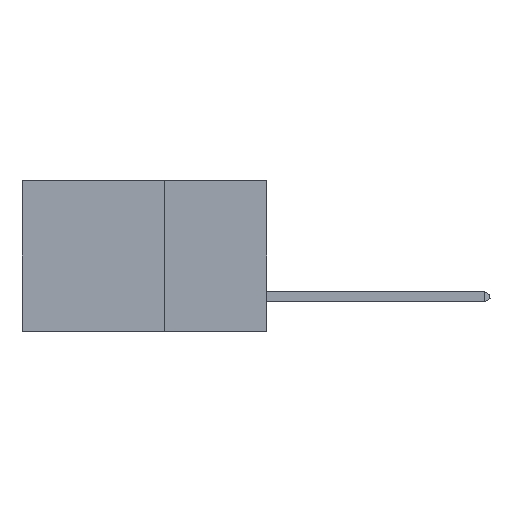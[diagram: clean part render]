
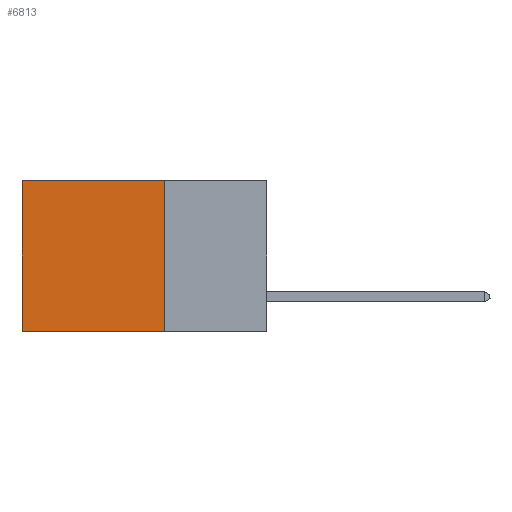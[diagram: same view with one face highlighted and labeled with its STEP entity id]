
A CAD part, left-side view. The second image highlights one B-rep face of the part: STEP entity #6813.
In plain terms, the highlighted planar face has unit normal (-1, 0, 0).
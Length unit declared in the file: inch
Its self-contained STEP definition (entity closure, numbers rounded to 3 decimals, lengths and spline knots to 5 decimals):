
#931 = LINE ( 'NONE', #12581, #39405 ) ;
#4380 = VERTEX_POINT ( 'NONE', #19535 ) ;
#6278 = CARTESIAN_POINT ( 'NONE',  ( 0.2875, 0.25, 0. ) ) ;
#6813 = ADVANCED_FACE ( 'NONE', ( #15004 ), #24079, .F. ) ;
#8796 = DIRECTION ( 'NONE',  ( 1., 0., 0. ) ) ;
#8923 = DIRECTION ( 'NONE',  ( 0., 0., -1. ) ) ;
#9191 = DIRECTION ( 'NONE',  ( 0., 0., -1. ) ) ;
#11655 = EDGE_LOOP ( 'NONE', ( #38648, #33947, #19372, #26252 ) ) ;
#12581 = CARTESIAN_POINT ( 'NONE',  ( 0.2875, 0.25, -0.37 ) ) ;
#12689 = CARTESIAN_POINT ( 'NONE',  ( 0.2875, 0.25, 0. ) ) ;
#12756 = DIRECTION ( 'NONE',  ( 0., 1., 0. ) ) ;
#14245 = CARTESIAN_POINT ( 'NONE',  ( 0.2875, 0.6, 0. ) ) ;
#14842 = CARTESIAN_POINT ( 'NONE',  ( 0.2875, 0.25, 0. ) ) ;
#15004 = FACE_OUTER_BOUND ( 'NONE', #11655, .T. ) ;
#16003 = LINE ( 'NONE', #12689, #34022 ) ;
#16936 = EDGE_CURVE ( 'NONE', #4380, #40893, #34545, .T. ) ;
#18085 = DIRECTION ( 'NONE',  ( 0., 1., 0. ) ) ;
#18658 = CARTESIAN_POINT ( 'NONE',  ( 0.2875, 0.6, -0.37 ) ) ;
#19372 = ORIENTED_EDGE ( 'NONE', *, *, #44187, .F. ) ;
#19535 = CARTESIAN_POINT ( 'NONE',  ( 0.2875, 0.6, 0. ) ) ;
#20780 = VERTEX_POINT ( 'NONE', #6278 ) ;
#21091 = EDGE_CURVE ( 'NONE', #44915, #40893, #931, .T. ) ;
#23468 = VECTOR ( 'NONE', #9191, 39.37008 ) ;
#24047 = LINE ( 'NONE', #14842, #30430 ) ;
#24079 = PLANE ( 'NONE',  #32971 ) ;
#26252 = ORIENTED_EDGE ( 'NONE', *, *, #33087, .T. ) ;
#27289 = CARTESIAN_POINT ( 'NONE',  ( 0.2875, 0.25, 0. ) ) ;
#30430 = VECTOR ( 'NONE', #18085, 39.37008 ) ;
#32971 = AXIS2_PLACEMENT_3D ( 'NONE', #27289, #8796, #46965 ) ;
#33087 = EDGE_CURVE ( 'NONE', #20780, #4380, #24047, .T. ) ;
#33947 = ORIENTED_EDGE ( 'NONE', *, *, #21091, .F. ) ;
#33986 = CARTESIAN_POINT ( 'NONE',  ( 0.2875, 0.25, -0.37 ) ) ;
#34022 = VECTOR ( 'NONE', #8923, 39.37008 ) ;
#34545 = LINE ( 'NONE', #14245, #23468 ) ;
#38648 = ORIENTED_EDGE ( 'NONE', *, *, #16936, .T. ) ;
#39405 = VECTOR ( 'NONE', #12756, 39.37008 ) ;
#40893 = VERTEX_POINT ( 'NONE', #18658 ) ;
#44187 = EDGE_CURVE ( 'NONE', #20780, #44915, #16003, .T. ) ;
#44915 = VERTEX_POINT ( 'NONE', #33986 ) ;
#46965 = DIRECTION ( 'NONE',  ( 0., 0., -1. ) ) ;
